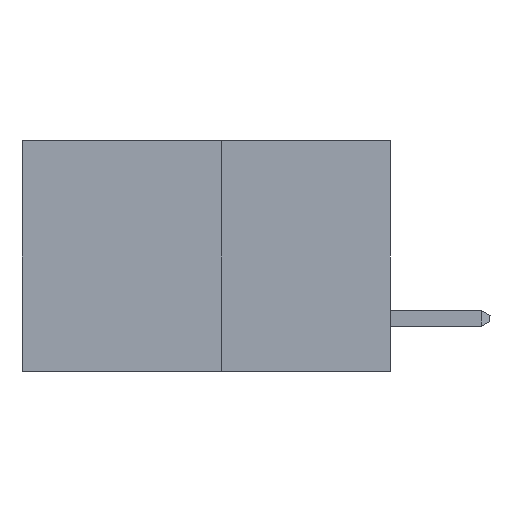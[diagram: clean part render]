
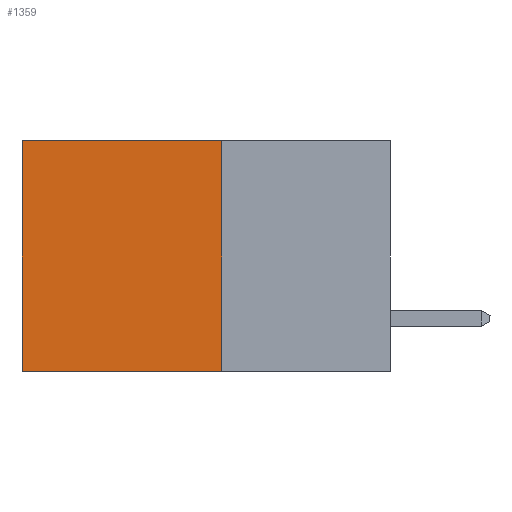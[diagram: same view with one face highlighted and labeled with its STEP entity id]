
A CAD part, left-side view. The second image highlights one B-rep face of the part: STEP entity #1359.
In plain terms, the highlighted planar face has unit normal (-1, 0, 0).
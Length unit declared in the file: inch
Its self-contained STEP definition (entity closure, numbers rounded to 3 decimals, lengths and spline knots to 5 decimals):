
#71 = LINE ( 'NONE', #7452, #11955 ) ;
#584 = DIRECTION ( 'NONE',  ( 0., 1., 0. ) ) ;
#994 = CARTESIAN_POINT ( 'NONE',  ( 0.277, 0.27, 0. ) ) ;
#1291 = EDGE_CURVE ( 'NONE', #9289, #3031, #71, .T. ) ;
#1359 = ADVANCED_FACE ( 'NONE', ( #12425 ), #6582, .F. ) ;
#1615 = CARTESIAN_POINT ( 'NONE',  ( 0.277, 0.59, -0.37 ) ) ;
#2282 = CARTESIAN_POINT ( 'NONE',  ( 0.277, 0.59, -0.37 ) ) ;
#2534 = DIRECTION ( 'NONE',  ( 0., 0., -1. ) ) ;
#2649 = EDGE_LOOP ( 'NONE', ( #10262, #8925, #11740, #7371 ) ) ;
#2667 = CARTESIAN_POINT ( 'NONE',  ( 0.277, 0.59, 0. ) ) ;
#2694 = DIRECTION ( 'NONE',  ( 1., 0., 0. ) ) ;
#3031 = VERTEX_POINT ( 'NONE', #2282 ) ;
#3534 = VECTOR ( 'NONE', #8819, 39.37008 ) ;
#3768 = EDGE_CURVE ( 'NONE', #14112, #9289, #8991, .T. ) ;
#3882 = CARTESIAN_POINT ( 'NONE',  ( 0.277, 0.27, 0. ) ) ;
#3957 = VECTOR ( 'NONE', #5159, 39.37008 ) ;
#4432 = CARTESIAN_POINT ( 'NONE',  ( 0.277, 0.27, -0.37 ) ) ;
#5159 = DIRECTION ( 'NONE',  ( 0., 1., 0. ) ) ;
#5553 = VERTEX_POINT ( 'NONE', #2667 ) ;
#6582 = PLANE ( 'NONE',  #12055 ) ;
#7371 = ORIENTED_EDGE ( 'NONE', *, *, #12631, .T. ) ;
#7452 = CARTESIAN_POINT ( 'NONE',  ( 0.277, 0.27, -0.37 ) ) ;
#8537 = CARTESIAN_POINT ( 'NONE',  ( 0.277, 0.27, -0.37 ) ) ;
#8654 = VECTOR ( 'NONE', #2534, 39.37008 ) ;
#8819 = DIRECTION ( 'NONE',  ( 0., 0., -1. ) ) ;
#8925 = ORIENTED_EDGE ( 'NONE', *, *, #1291, .F. ) ;
#8944 = CARTESIAN_POINT ( 'NONE',  ( 0.277, 0.27, -0.37 ) ) ;
#8991 = LINE ( 'NONE', #4432, #8654 ) ;
#9289 = VERTEX_POINT ( 'NONE', #8537 ) ;
#10262 = ORIENTED_EDGE ( 'NONE', *, *, #13754, .T. ) ;
#11740 = ORIENTED_EDGE ( 'NONE', *, *, #3768, .F. ) ;
#11811 = LINE ( 'NONE', #1615, #3534 ) ;
#11955 = VECTOR ( 'NONE', #584, 39.37008 ) ;
#12055 = AXIS2_PLACEMENT_3D ( 'NONE', #8944, #2694, #13798 ) ;
#12425 = FACE_OUTER_BOUND ( 'NONE', #2649, .T. ) ;
#12631 = EDGE_CURVE ( 'NONE', #14112, #5553, #13364, .T. ) ;
#13364 = LINE ( 'NONE', #3882, #3957 ) ;
#13754 = EDGE_CURVE ( 'NONE', #5553, #3031, #11811, .T. ) ;
#13798 = DIRECTION ( 'NONE',  ( 0., 0., -1. ) ) ;
#14112 = VERTEX_POINT ( 'NONE', #994 ) ;
